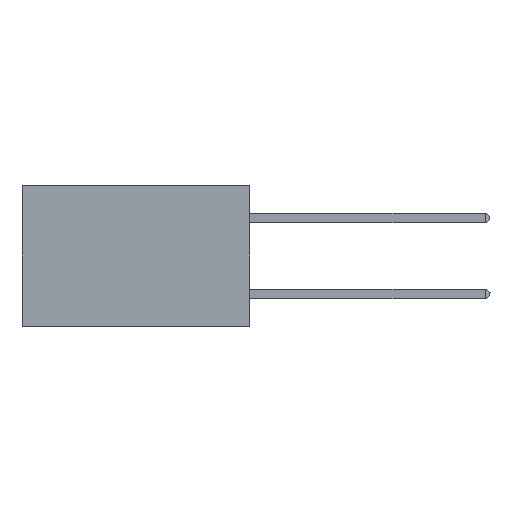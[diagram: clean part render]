
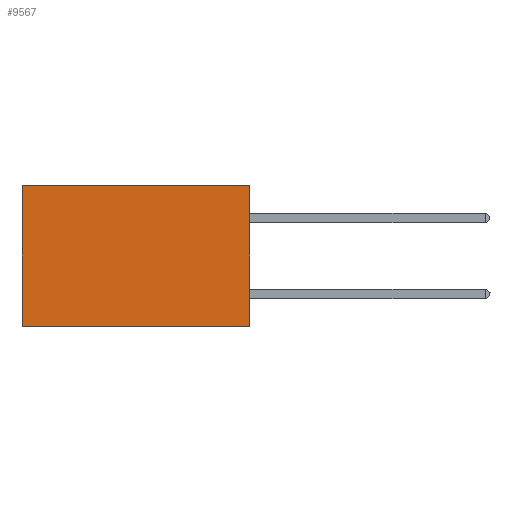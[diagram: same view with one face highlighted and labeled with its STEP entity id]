
A CAD part, left-side view. The second image highlights one B-rep face of the part: STEP entity #9567.
In plain terms, the highlighted planar face has unit normal (-1, 0, 0).
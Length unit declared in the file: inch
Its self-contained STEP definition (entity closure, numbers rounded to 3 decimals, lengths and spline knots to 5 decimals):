
#7 = ORIENTED_EDGE ( 'NONE', *, *, #24703, .F. ) ;
#652 = DIRECTION ( 'NONE',  ( 0., 1., 0. ) ) ;
#1789 = ORIENTED_EDGE ( 'NONE', *, *, #32305, .T. ) ;
#2496 = CARTESIAN_POINT ( 'NONE',  ( 0.2875, 0.6, -0.37 ) ) ;
#3294 = CARTESIAN_POINT ( 'NONE',  ( 0.2875, 0.6, 0. ) ) ;
#4632 = AXIS2_PLACEMENT_3D ( 'NONE', #13991, #8418, #26141 ) ;
#5395 = EDGE_CURVE ( 'NONE', #30225, #21377, #36420, .T. ) ;
#6261 = ORIENTED_EDGE ( 'NONE', *, *, #5395, .T. ) ;
#6286 = VECTOR ( 'NONE', #27097, 39.37008 ) ;
#7617 = CARTESIAN_POINT ( 'NONE',  ( 0.2875, 0., 0. ) ) ;
#8418 = DIRECTION ( 'NONE',  ( 1., 0., 0. ) ) ;
#9567 = ADVANCED_FACE ( 'NONE', ( #27772 ), #11611, .F. ) ;
#11393 = VECTOR ( 'NONE', #34496, 39.37008 ) ;
#11611 = PLANE ( 'NONE',  #4632 ) ;
#13042 = CARTESIAN_POINT ( 'NONE',  ( 0.2875, 0., 0. ) ) ;
#13257 = VERTEX_POINT ( 'NONE', #2496 ) ;
#13991 = CARTESIAN_POINT ( 'NONE',  ( 0.2875, 0., 0. ) ) ;
#14247 = CARTESIAN_POINT ( 'NONE',  ( 0.2875, 0.6, 0. ) ) ;
#14595 = CARTESIAN_POINT ( 'NONE',  ( 0.2875, 0., -0.37 ) ) ;
#17402 = VERTEX_POINT ( 'NONE', #29465 ) ;
#18128 = LINE ( 'NONE', #14595, #35055 ) ;
#21377 = VERTEX_POINT ( 'NONE', #14247 ) ;
#22773 = CARTESIAN_POINT ( 'NONE',  ( 0.2875, 0., 0. ) ) ;
#22913 = LINE ( 'NONE', #3294, #11393 ) ;
#24463 = DIRECTION ( 'NONE',  ( 0., 0., -1. ) ) ;
#24703 = EDGE_CURVE ( 'NONE', #30225, #17402, #33415, .T. ) ;
#25551 = ORIENTED_EDGE ( 'NONE', *, *, #26209, .F. ) ;
#25879 = VECTOR ( 'NONE', #24463, 39.37008 ) ;
#26141 = DIRECTION ( 'NONE',  ( 0., 0., -1. ) ) ;
#26209 = EDGE_CURVE ( 'NONE', #17402, #13257, #18128, .T. ) ;
#27097 = DIRECTION ( 'NONE',  ( 0., 1., 0. ) ) ;
#27772 = FACE_OUTER_BOUND ( 'NONE', #36174, .T. ) ;
#29465 = CARTESIAN_POINT ( 'NONE',  ( 0.2875, 0., -0.37 ) ) ;
#30225 = VERTEX_POINT ( 'NONE', #22773 ) ;
#32305 = EDGE_CURVE ( 'NONE', #21377, #13257, #22913, .T. ) ;
#33415 = LINE ( 'NONE', #13042, #25879 ) ;
#34496 = DIRECTION ( 'NONE',  ( 0., 0., -1. ) ) ;
#35055 = VECTOR ( 'NONE', #652, 39.37008 ) ;
#36174 = EDGE_LOOP ( 'NONE', ( #1789, #25551, #7, #6261 ) ) ;
#36420 = LINE ( 'NONE', #7617, #6286 ) ;
